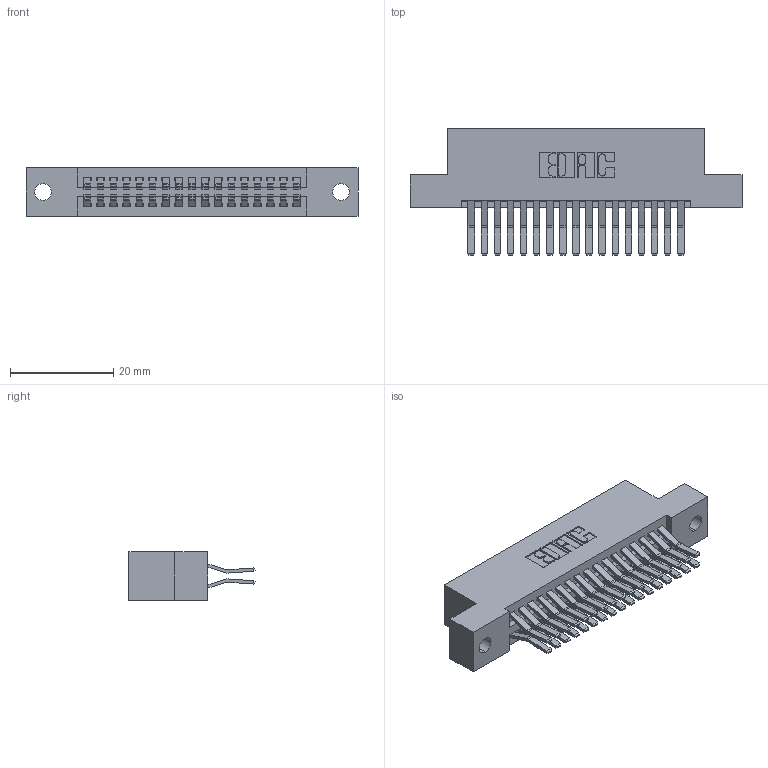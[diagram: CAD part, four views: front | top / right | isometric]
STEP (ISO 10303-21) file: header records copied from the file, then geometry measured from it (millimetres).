
FILE_DESCRIPTION (( 'STEP AP203' ), '1' );
FILE_NAME ('395-034-560-202.STEP', '2019-10-17T18:41:44', ( '' ), ( '' ), 'SwSTEP 2.0', 'SolidWorks 2016', '' );
FILE_SCHEMA (( 'CONFIG_CONTROL_DESIGN' ));
Length unit declared in the file: inch
Products named in the file (3): 345 Part_Flush Mounting Lugs - 0.128 Dia; 345-292-001_560 Tail; 395-034-560-202
Assembly tree (35 placements, depth 2):
  395-034-560-202
    345 Part_Flush Mounting Lugs - 0.128 Dia
    345-292-001_560 Tail  x34
Bounding box: 64.39 x 24.45 x 9.4 mm (x, y, z)
Volume: 6208.9 mm3; surface area: 8994.1 mm2
Topology: 35 solids, 35 shells, 1894 faces, 5611 edges, 3694 vertices
Faces by surface type: plane 1202, cylinder 692
Entity records: 16795 total; most frequent: CARTESIAN_POINT 2840, ORIENTED_EDGE 2774, DIRECTION 2539, EDGE_CURVE 1387, VECTOR 1183, LINE 1183, VERTEX_POINT 922, AXIS2_PLACEMENT_3D 678
